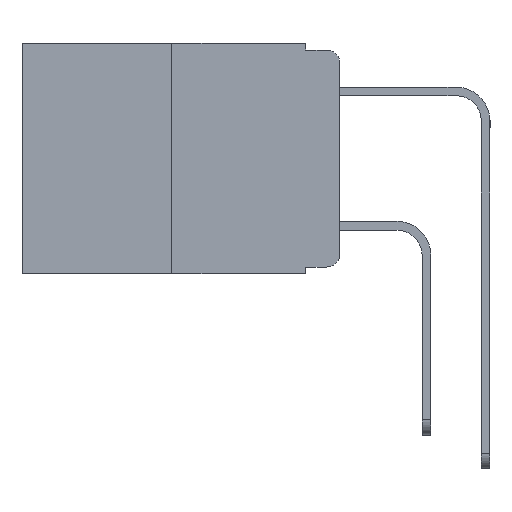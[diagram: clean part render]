
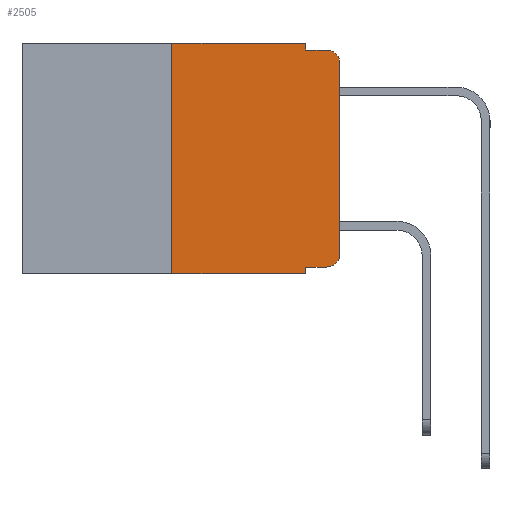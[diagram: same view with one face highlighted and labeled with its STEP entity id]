
A CAD part, left-side view. The second image highlights one B-rep face of the part: STEP entity #2505.
In plain terms, the highlighted planar face has unit normal (-1, 0, 0).
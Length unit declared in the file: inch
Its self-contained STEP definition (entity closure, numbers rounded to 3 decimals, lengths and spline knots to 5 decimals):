
#12 = AXIS2_PLACEMENT_3D ( 'NONE', #9076, #12636, #8703 ) ;
#25 = ORIENTED_EDGE ( 'NONE', *, *, #7618, .T. ) ;
#151 = CARTESIAN_POINT ( 'NONE',  ( 0., 0.02, -0.01 ) ) ;
#345 = LINE ( 'NONE', #12466, #8640 ) ;
#1113 = CARTESIAN_POINT ( 'NONE',  ( 0., 0.051, 0. ) ) ;
#1128 = ORIENTED_EDGE ( 'NONE', *, *, #3987, .F. ) ;
#1386 = ORIENTED_EDGE ( 'NONE', *, *, #5089, .F. ) ;
#1520 = ORIENTED_EDGE ( 'NONE', *, *, #8352, .T. ) ;
#1768 = CIRCLE ( 'NONE', #2589, 0.02 ) ;
#1815 = EDGE_CURVE ( 'NONE', #4370, #6384, #8236, .T. ) ;
#1993 = DIRECTION ( 'NONE',  ( 0., -1., 0. ) ) ;
#1999 = CARTESIAN_POINT ( 'NONE',  ( 0., 0.051, -0.333 ) ) ;
#2024 = DIRECTION ( 'NONE',  ( -1., 0., 0. ) ) ;
#2471 = VERTEX_POINT ( 'NONE', #10487 ) ;
#2505 = ADVANCED_FACE ( 'NONE', ( #5492 ), #11475, .F. ) ;
#2530 = EDGE_CURVE ( 'NONE', #2471, #4370, #10180, .T. ) ;
#2571 = ORIENTED_EDGE ( 'NONE', *, *, #4716, .F. ) ;
#2589 = AXIS2_PLACEMENT_3D ( 'NONE', #8514, #2024, #9564 ) ;
#2851 = VECTOR ( 'NONE', #10903, 39.37008 ) ;
#3046 = ORIENTED_EDGE ( 'NONE', *, *, #1815, .T. ) ;
#3074 = DIRECTION ( 'NONE',  ( 0., -1., 0. ) ) ;
#3194 = EDGE_LOOP ( 'NONE', ( #1520, #25, #4665, #2571, #1386, #1128, #12547, #11419, #12425, #3046 ) ) ;
#3326 = VERTEX_POINT ( 'NONE', #1113 ) ;
#3440 = EDGE_CURVE ( 'NONE', #12599, #3701, #12762, .T. ) ;
#3701 = VERTEX_POINT ( 'NONE', #9387 ) ;
#3987 = EDGE_CURVE ( 'NONE', #12599, #6531, #13056, .T. ) ;
#4117 = DIRECTION ( 'NONE',  ( 0., 0., -1. ) ) ;
#4370 = VERTEX_POINT ( 'NONE', #10441 ) ;
#4402 = VECTOR ( 'NONE', #6593, 39.37008 ) ;
#4665 = ORIENTED_EDGE ( 'NONE', *, *, #6167, .F. ) ;
#4716 = EDGE_CURVE ( 'NONE', #3326, #8828, #5072, .T. ) ;
#4821 = CARTESIAN_POINT ( 'NONE',  ( 0., 0., -0.03 ) ) ;
#5072 = LINE ( 'NONE', #11896, #2851 ) ;
#5089 = EDGE_CURVE ( 'NONE', #6531, #3326, #8946, .T. ) ;
#5492 = FACE_OUTER_BOUND ( 'NONE', #3194, .T. ) ;
#6140 = DIRECTION ( 'NONE',  ( 0., 0., 1. ) ) ;
#6167 = EDGE_CURVE ( 'NONE', #8828, #12603, #12992, .T. ) ;
#6268 = DIRECTION ( 'NONE',  ( 0., 0., -1. ) ) ;
#6384 = VERTEX_POINT ( 'NONE', #7316 ) ;
#6450 = CARTESIAN_POINT ( 'NONE',  ( 0., 0.25, 0. ) ) ;
#6503 = VECTOR ( 'NONE', #6140, 39.37008 ) ;
#6531 = VERTEX_POINT ( 'NONE', #6450 ) ;
#6593 = DIRECTION ( 'NONE',  ( 0., 0., 1. ) ) ;
#6799 = DIRECTION ( 'NONE',  ( 0., -1., 0. ) ) ;
#6986 = CARTESIAN_POINT ( 'NONE',  ( 0., 0.051, -0.01 ) ) ;
#6990 = DIRECTION ( 'NONE',  ( 0., -1., 0. ) ) ;
#7316 = CARTESIAN_POINT ( 'NONE',  ( 0., 0., -0.313 ) ) ;
#7360 = VECTOR ( 'NONE', #3074, 39.37008 ) ;
#7398 = CARTESIAN_POINT ( 'NONE',  ( 0., 0.473, 0. ) ) ;
#7618 = EDGE_CURVE ( 'NONE', #9985, #12603, #1768, .T. ) ;
#8236 = CIRCLE ( 'NONE', #12, 0.02 ) ;
#8352 = EDGE_CURVE ( 'NONE', #6384, #9985, #9377, .T. ) ;
#8514 = CARTESIAN_POINT ( 'NONE',  ( 0., 0.02, -0.03 ) ) ;
#8640 = VECTOR ( 'NONE', #6268, 39.37008 ) ;
#8703 = DIRECTION ( 'NONE',  ( 0., 0., -1. ) ) ;
#8828 = VERTEX_POINT ( 'NONE', #6986 ) ;
#8902 = AXIS2_PLACEMENT_3D ( 'NONE', #9464, #10535, #4117 ) ;
#8946 = LINE ( 'NONE', #7398, #11629 ) ;
#9076 = CARTESIAN_POINT ( 'NONE',  ( 0., 0.02, -0.313 ) ) ;
#9377 = LINE ( 'NONE', #10382, #6503 ) ;
#9387 = CARTESIAN_POINT ( 'NONE',  ( 0., 0.051, -0.343 ) ) ;
#9464 = CARTESIAN_POINT ( 'NONE',  ( 0., 0.473, 0. ) ) ;
#9564 = DIRECTION ( 'NONE',  ( 0., 0., -1. ) ) ;
#9813 = CARTESIAN_POINT ( 'NONE',  ( 0., 0.25, -0.343 ) ) ;
#9985 = VERTEX_POINT ( 'NONE', #4821 ) ;
#10137 = VECTOR ( 'NONE', #6799, 39.37008 ) ;
#10180 = LINE ( 'NONE', #1999, #7360 ) ;
#10382 = CARTESIAN_POINT ( 'NONE',  ( 0., 0., 0. ) ) ;
#10441 = CARTESIAN_POINT ( 'NONE',  ( 0., 0.02, -0.333 ) ) ;
#10487 = CARTESIAN_POINT ( 'NONE',  ( 0., 0.051, -0.333 ) ) ;
#10535 = DIRECTION ( 'NONE',  ( 1., 0., 0. ) ) ;
#10791 = CARTESIAN_POINT ( 'NONE',  ( 0., 0.25, 0. ) ) ;
#10903 = DIRECTION ( 'NONE',  ( 0., 0., -1. ) ) ;
#11419 = ORIENTED_EDGE ( 'NONE', *, *, #12405, .F. ) ;
#11475 = PLANE ( 'NONE',  #8902 ) ;
#11629 = VECTOR ( 'NONE', #1993, 39.37008 ) ;
#11896 = CARTESIAN_POINT ( 'NONE',  ( 0., 0.051, 0. ) ) ;
#11965 = CARTESIAN_POINT ( 'NONE',  ( 0., 0.473, -0.343 ) ) ;
#12139 = CARTESIAN_POINT ( 'NONE',  ( 0., 0.051, -0.01 ) ) ;
#12405 = EDGE_CURVE ( 'NONE', #2471, #3701, #345, .T. ) ;
#12425 = ORIENTED_EDGE ( 'NONE', *, *, #2530, .T. ) ;
#12466 = CARTESIAN_POINT ( 'NONE',  ( 0., 0.051, 0. ) ) ;
#12547 = ORIENTED_EDGE ( 'NONE', *, *, #3440, .T. ) ;
#12599 = VERTEX_POINT ( 'NONE', #9813 ) ;
#12603 = VERTEX_POINT ( 'NONE', #151 ) ;
#12636 = DIRECTION ( 'NONE',  ( -1., 0., 0. ) ) ;
#12762 = LINE ( 'NONE', #11965, #10137 ) ;
#12992 = LINE ( 'NONE', #12139, #13305 ) ;
#13056 = LINE ( 'NONE', #10791, #4402 ) ;
#13305 = VECTOR ( 'NONE', #6990, 39.37008 ) ;
